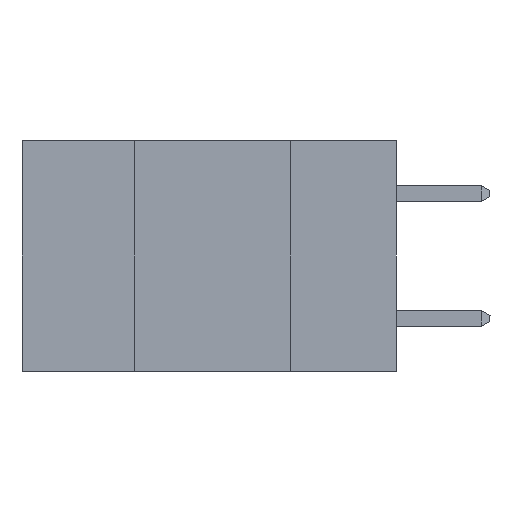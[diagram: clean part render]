
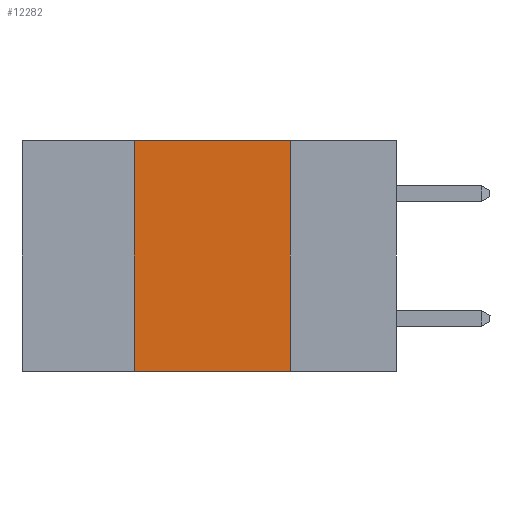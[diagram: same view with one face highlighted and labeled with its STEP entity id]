
A CAD part, left-side view. The second image highlights one B-rep face of the part: STEP entity #12282.
In plain terms, the highlighted planar face has unit normal (-1, 0, 0).
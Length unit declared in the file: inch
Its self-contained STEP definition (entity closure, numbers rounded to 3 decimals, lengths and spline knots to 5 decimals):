
#358 = VERTEX_POINT ( 'NONE', #8061 ) ;
#978 = VECTOR ( 'NONE', #8255, 39.37008 ) ;
#1205 = VERTEX_POINT ( 'NONE', #14584 ) ;
#2966 = CARTESIAN_POINT ( 'NONE',  ( 0., 0.17, 0. ) ) ;
#3220 = EDGE_CURVE ( 'NONE', #7957, #358, #4341, .T. ) ;
#4271 = VECTOR ( 'NONE', #13326, 39.37008 ) ;
#4341 = LINE ( 'NONE', #8700, #8402 ) ;
#4359 = ORIENTED_EDGE ( 'NONE', *, *, #3220, .F. ) ;
#4568 = DIRECTION ( 'NONE',  ( 0., 0., -1. ) ) ;
#4885 = CARTESIAN_POINT ( 'NONE',  ( 0., 0.42, 0. ) ) ;
#4895 = EDGE_LOOP ( 'NONE', ( #11605, #4359, #6891, #14513 ) ) ;
#5394 = DIRECTION ( 'NONE',  ( 0., -1., 0. ) ) ;
#5710 = LINE ( 'NONE', #9910, #4271 ) ;
#5731 = DIRECTION ( 'NONE',  ( 1., 0., 0. ) ) ;
#6053 = EDGE_CURVE ( 'NONE', #7211, #1205, #5710, .T. ) ;
#6688 = CARTESIAN_POINT ( 'NONE',  ( 0., 0.42, -0.37 ) ) ;
#6774 = CARTESIAN_POINT ( 'NONE',  ( 0., 0.6, 0. ) ) ;
#6891 = ORIENTED_EDGE ( 'NONE', *, *, #11271, .F. ) ;
#7211 = VERTEX_POINT ( 'NONE', #6688 ) ;
#7957 = VERTEX_POINT ( 'NONE', #11709 ) ;
#8061 = CARTESIAN_POINT ( 'NONE',  ( 0., 0.17, 0. ) ) ;
#8255 = DIRECTION ( 'NONE',  ( 0., 0., 1. ) ) ;
#8402 = VECTOR ( 'NONE', #5394, 39.37008 ) ;
#8629 = AXIS2_PLACEMENT_3D ( 'NONE', #6774, #5731, #4568 ) ;
#8700 = CARTESIAN_POINT ( 'NONE',  ( 0., 0.6, 0. ) ) ;
#8800 = VECTOR ( 'NONE', #14377, 39.37008 ) ;
#9596 = EDGE_CURVE ( 'NONE', #358, #1205, #11269, .T. ) ;
#9910 = CARTESIAN_POINT ( 'NONE',  ( 0., 0.6, -0.37 ) ) ;
#11269 = LINE ( 'NONE', #2966, #8800 ) ;
#11271 = EDGE_CURVE ( 'NONE', #7211, #7957, #14262, .T. ) ;
#11290 = PLANE ( 'NONE',  #8629 ) ;
#11605 = ORIENTED_EDGE ( 'NONE', *, *, #9596, .F. ) ;
#11709 = CARTESIAN_POINT ( 'NONE',  ( 0., 0.42, 0. ) ) ;
#12282 = ADVANCED_FACE ( 'NONE', ( #14051 ), #11290, .F. ) ;
#13326 = DIRECTION ( 'NONE',  ( 0., -1., 0. ) ) ;
#14051 = FACE_OUTER_BOUND ( 'NONE', #4895, .T. ) ;
#14262 = LINE ( 'NONE', #4885, #978 ) ;
#14377 = DIRECTION ( 'NONE',  ( 0., 0., -1. ) ) ;
#14513 = ORIENTED_EDGE ( 'NONE', *, *, #6053, .T. ) ;
#14584 = CARTESIAN_POINT ( 'NONE',  ( 0., 0.17, -0.37 ) ) ;
